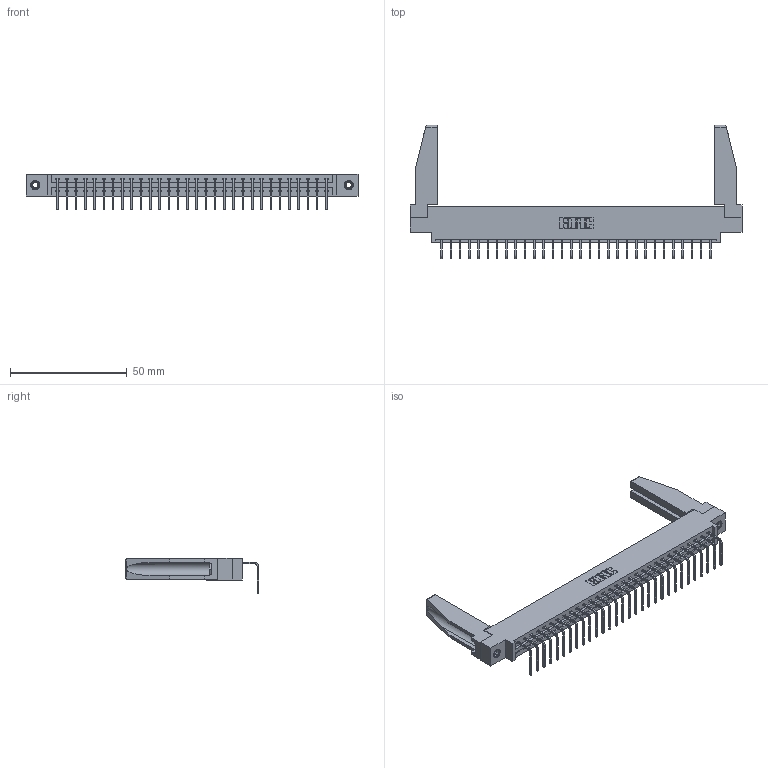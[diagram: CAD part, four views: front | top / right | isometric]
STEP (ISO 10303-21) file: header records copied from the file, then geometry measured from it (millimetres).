
FILE_DESCRIPTION (( 'STEP AP203' ), '1' );
FILE_NAME ('387-030-558-678.STEP', '2019-10-07T19:37:32', ( '' ), ( '' ), 'SwSTEP 2.0', 'SolidWorks 2016', '' );
FILE_SCHEMA (( 'CONFIG_CONTROL_DESIGN' ));
Length unit declared in the file: inch
Products named in the file (5): 345-250-001_345-250-001-102; 387-030-558-678; 337 Part_0.170 Offset - 0.156 Dia-TI; 345-292-001_558 Tail - 2; 307-220-078
Assembly tree (35 placements, depth 2):
  387-030-558-678
    337 Part_0.170 Offset - 0.156 Dia-TI
    345-292-001_558 Tail - 2  x30
    345-250-001_345-250-001-102  x2
    307-220-078  x2
Bounding box: 141.88 x 56.96 x 15.37 mm (x, y, z)
Volume: 18572.1 mm3; surface area: 19545.8 mm2
Topology: 35 solids, 35 shells, 2168 faces, 6473 edges, 4266 vertices
Faces by surface type: plane 1598, cylinder 554, cone 12, torus 4
Entity records: 26508 total; most frequent: CARTESIAN_POINT 4610, ORIENTED_EDGE 4532, DIRECTION 3914, EDGE_CURVE 2266, LINE 2100, VECTOR 2100, VERTEX_POINT 1504, AXIS2_PLACEMENT_3D 907
